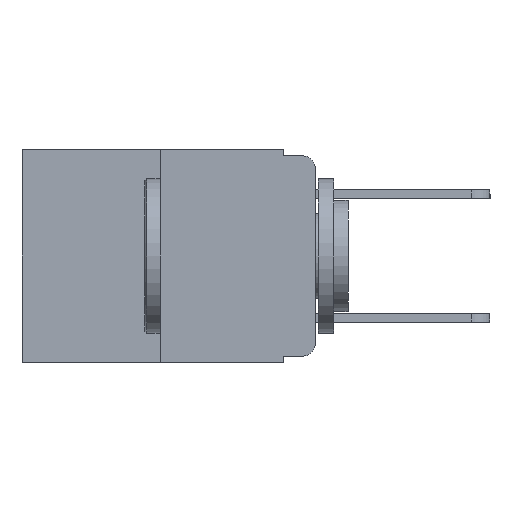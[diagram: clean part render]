
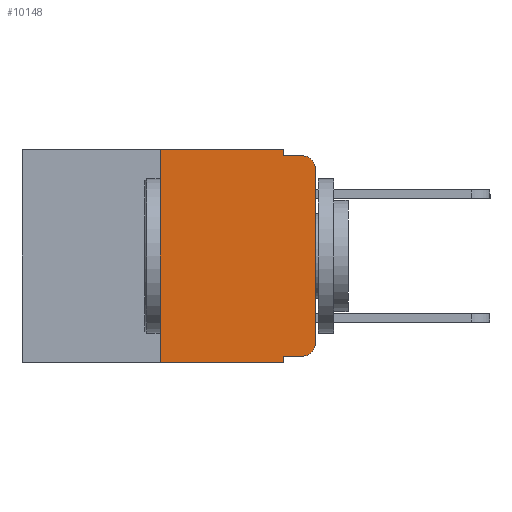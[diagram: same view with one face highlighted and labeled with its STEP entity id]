
A CAD part, left-side view. The second image highlights one B-rep face of the part: STEP entity #10148.
In plain terms, the highlighted planar face has unit normal (-1, 0, 0).
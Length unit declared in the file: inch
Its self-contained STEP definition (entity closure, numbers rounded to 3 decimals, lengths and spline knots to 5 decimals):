
#58 = CARTESIAN_POINT ( 'NONE',  ( 0., 0.051, 0. ) ) ;
#429 = CARTESIAN_POINT ( 'NONE',  ( 0., 0.25, 0. ) ) ;
#553 = ORIENTED_EDGE ( 'NONE', *, *, #3023, .F. ) ;
#1219 = VECTOR ( 'NONE', #15393, 39.37008 ) ;
#1244 = DIRECTION ( 'NONE',  ( 0., 0., -1. ) ) ;
#1325 = ORIENTED_EDGE ( 'NONE', *, *, #13971, .T. ) ;
#1425 = DIRECTION ( 'NONE',  ( 0., 0., -1. ) ) ;
#1722 = CARTESIAN_POINT ( 'NONE',  ( 0., 0.051, 0. ) ) ;
#1780 = ORIENTED_EDGE ( 'NONE', *, *, #15081, .F. ) ;
#1783 = EDGE_CURVE ( 'NONE', #8550, #2617, #2870, .T. ) ;
#1903 = ORIENTED_EDGE ( 'NONE', *, *, #12763, .F. ) ;
#1925 = LINE ( 'NONE', #15343, #5296 ) ;
#2229 = EDGE_CURVE ( 'NONE', #9721, #2617, #11534, .T. ) ;
#2328 = EDGE_CURVE ( 'NONE', #4442, #5038, #5741, .T. ) ;
#2378 = VECTOR ( 'NONE', #15185, 39.37008 ) ;
#2617 = VERTEX_POINT ( 'NONE', #16528 ) ;
#2870 = LINE ( 'NONE', #4837, #6137 ) ;
#3023 = EDGE_CURVE ( 'NONE', #6882, #8751, #1925, .T. ) ;
#3251 = CARTESIAN_POINT ( 'NONE',  ( 0., 0., -0.313 ) ) ;
#3424 = ORIENTED_EDGE ( 'NONE', *, *, #2328, .T. ) ;
#3445 = ORIENTED_EDGE ( 'NONE', *, *, #1783, .F. ) ;
#3473 = EDGE_CURVE ( 'NONE', #14413, #9721, #16171, .T. ) ;
#3480 = VERTEX_POINT ( 'NONE', #7168 ) ;
#3531 = AXIS2_PLACEMENT_3D ( 'NONE', #11830, #3812, #13100 ) ;
#3812 = DIRECTION ( 'NONE',  ( -1., 0., 0. ) ) ;
#4129 = DIRECTION ( 'NONE',  ( 1., 0., 0. ) ) ;
#4278 = CARTESIAN_POINT ( 'NONE',  ( 0., 0.051, -0.333 ) ) ;
#4442 = VERTEX_POINT ( 'NONE', #4278 ) ;
#4837 = CARTESIAN_POINT ( 'NONE',  ( 0., 0.051, -0.01 ) ) ;
#5020 = LINE ( 'NONE', #1722, #8188 ) ;
#5038 = VERTEX_POINT ( 'NONE', #12360 ) ;
#5296 = VECTOR ( 'NONE', #15637, 39.37008 ) ;
#5501 = CARTESIAN_POINT ( 'NONE',  ( 0., 0.25, -0.343 ) ) ;
#5741 = LINE ( 'NONE', #12894, #12341 ) ;
#5880 = VECTOR ( 'NONE', #10892, 39.37008 ) ;
#6055 = CARTESIAN_POINT ( 'NONE',  ( 0., 0., -0.03 ) ) ;
#6137 = VECTOR ( 'NONE', #15822, 39.37008 ) ;
#6321 = CARTESIAN_POINT ( 'NONE',  ( 0., 0.473, -0.343 ) ) ;
#6519 = LINE ( 'NONE', #13933, #2378 ) ;
#6882 = VERTEX_POINT ( 'NONE', #429 ) ;
#6976 = CARTESIAN_POINT ( 'NONE',  ( 0., 0.051, -0.01 ) ) ;
#7168 = CARTESIAN_POINT ( 'NONE',  ( 0., 0.051, -0.343 ) ) ;
#7865 = LINE ( 'NONE', #6321, #1219 ) ;
#8188 = VECTOR ( 'NONE', #9963, 39.37008 ) ;
#8452 = ORIENTED_EDGE ( 'NONE', *, *, #2229, .T. ) ;
#8493 = VERTEX_POINT ( 'NONE', #5501 ) ;
#8550 = VERTEX_POINT ( 'NONE', #6976 ) ;
#8751 = VERTEX_POINT ( 'NONE', #58 ) ;
#9452 = DIRECTION ( 'NONE',  ( 0., -1., 0. ) ) ;
#9509 = PLANE ( 'NONE',  #16377 ) ;
#9721 = VERTEX_POINT ( 'NONE', #6055 ) ;
#9963 = DIRECTION ( 'NONE',  ( 0., 0., -1. ) ) ;
#9976 = ORIENTED_EDGE ( 'NONE', *, *, #10853, .T. ) ;
#10148 = ADVANCED_FACE ( 'NONE', ( #14642 ), #9509, .F. ) ;
#10282 = ORIENTED_EDGE ( 'NONE', *, *, #3473, .T. ) ;
#10360 = ORIENTED_EDGE ( 'NONE', *, *, #11889, .F. ) ;
#10811 = CARTESIAN_POINT ( 'NONE',  ( 0., 0.473, 0. ) ) ;
#10853 = EDGE_CURVE ( 'NONE', #5038, #14413, #10869, .T. ) ;
#10869 = CIRCLE ( 'NONE', #3531, 0.02 ) ;
#10892 = DIRECTION ( 'NONE',  ( 0., 0., 1. ) ) ;
#10995 = VECTOR ( 'NONE', #1244, 39.37008 ) ;
#11534 = CIRCLE ( 'NONE', #15993, 0.02 ) ;
#11584 = CARTESIAN_POINT ( 'NONE',  ( 0., 0., 0. ) ) ;
#11830 = CARTESIAN_POINT ( 'NONE',  ( 0., 0.02, -0.313 ) ) ;
#11889 = EDGE_CURVE ( 'NONE', #8751, #8550, #5020, .T. ) ;
#12219 = LINE ( 'NONE', #14644, #10995 ) ;
#12341 = VECTOR ( 'NONE', #9452, 39.37008 ) ;
#12360 = CARTESIAN_POINT ( 'NONE',  ( 0., 0.02, -0.333 ) ) ;
#12763 = EDGE_CURVE ( 'NONE', #4442, #3480, #12219, .T. ) ;
#12894 = CARTESIAN_POINT ( 'NONE',  ( 0., 0.051, -0.333 ) ) ;
#13100 = DIRECTION ( 'NONE',  ( 0., 0., -1. ) ) ;
#13389 = DIRECTION ( 'NONE',  ( 0., 0., -1. ) ) ;
#13933 = CARTESIAN_POINT ( 'NONE',  ( 0., 0.25, 0. ) ) ;
#13971 = EDGE_CURVE ( 'NONE', #8493, #3480, #7865, .T. ) ;
#14413 = VERTEX_POINT ( 'NONE', #3251 ) ;
#14642 = FACE_OUTER_BOUND ( 'NONE', #16356, .T. ) ;
#14644 = CARTESIAN_POINT ( 'NONE',  ( 0., 0.051, 0. ) ) ;
#15081 = EDGE_CURVE ( 'NONE', #8493, #6882, #6519, .T. ) ;
#15185 = DIRECTION ( 'NONE',  ( 0., 0., 1. ) ) ;
#15343 = CARTESIAN_POINT ( 'NONE',  ( 0., 0.473, 0. ) ) ;
#15393 = DIRECTION ( 'NONE',  ( 0., -1., 0. ) ) ;
#15637 = DIRECTION ( 'NONE',  ( 0., -1., 0. ) ) ;
#15676 = DIRECTION ( 'NONE',  ( -1., 0., 0. ) ) ;
#15822 = DIRECTION ( 'NONE',  ( 0., -1., 0. ) ) ;
#15993 = AXIS2_PLACEMENT_3D ( 'NONE', #16531, #15676, #1425 ) ;
#16171 = LINE ( 'NONE', #11584, #5880 ) ;
#16356 = EDGE_LOOP ( 'NONE', ( #10282, #8452, #3445, #10360, #553, #1780, #1325, #1903, #3424, #9976 ) ) ;
#16377 = AXIS2_PLACEMENT_3D ( 'NONE', #10811, #4129, #13389 ) ;
#16528 = CARTESIAN_POINT ( 'NONE',  ( 0., 0.02, -0.01 ) ) ;
#16531 = CARTESIAN_POINT ( 'NONE',  ( 0., 0.02, -0.03 ) ) ;
